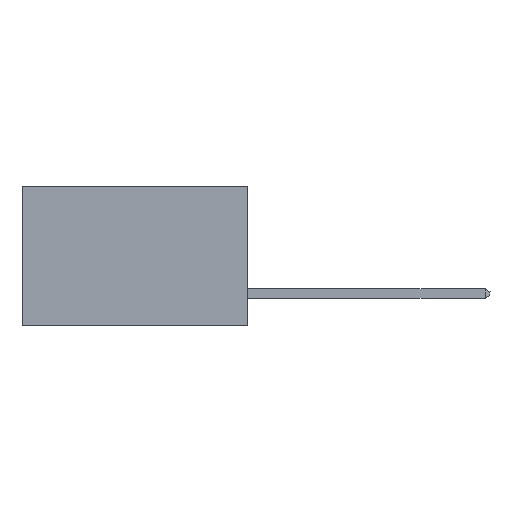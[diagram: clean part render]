
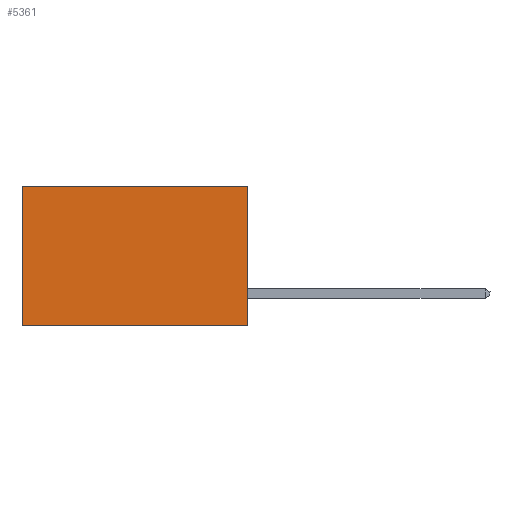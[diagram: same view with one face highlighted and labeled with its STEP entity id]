
A CAD part, left-side view. The second image highlights one B-rep face of the part: STEP entity #5361.
In plain terms, the highlighted planar face has unit normal (-1, 0, 0).
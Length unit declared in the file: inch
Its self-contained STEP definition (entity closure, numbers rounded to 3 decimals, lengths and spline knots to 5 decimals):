
#137 = EDGE_CURVE ( 'NONE', #7406, #227, #6344, .T. ) ;
#227 = VERTEX_POINT ( 'NONE', #5044 ) ;
#531 = CARTESIAN_POINT ( 'NONE',  ( 0.2615, 0.6, -0.37 ) ) ;
#715 = VECTOR ( 'NONE', #3175, 39.37008 ) ;
#822 = FACE_OUTER_BOUND ( 'NONE', #2043, .T. ) ;
#866 = VECTOR ( 'NONE', #8240, 39.37008 ) ;
#924 = ORIENTED_EDGE ( 'NONE', *, *, #137, .T. ) ;
#1146 = DIRECTION ( 'NONE',  ( 0., 1., 0. ) ) ;
#2043 = EDGE_LOOP ( 'NONE', ( #2177, #7409, #5523, #924 ) ) ;
#2177 = ORIENTED_EDGE ( 'NONE', *, *, #7890, .T. ) ;
#3007 = DIRECTION ( 'NONE',  ( 1., 0., 0. ) ) ;
#3175 = DIRECTION ( 'NONE',  ( 0., 0., -1. ) ) ;
#3201 = VECTOR ( 'NONE', #1146, 39.37008 ) ;
#4144 = CARTESIAN_POINT ( 'NONE',  ( 0.2615, 0., -0.37 ) ) ;
#4199 = VERTEX_POINT ( 'NONE', #5785 ) ;
#4618 = VECTOR ( 'NONE', #5422, 39.37008 ) ;
#5044 = CARTESIAN_POINT ( 'NONE',  ( 0.2615, 0.6, 0. ) ) ;
#5123 = CARTESIAN_POINT ( 'NONE',  ( 0.2615, 0., 0. ) ) ;
#5172 = CARTESIAN_POINT ( 'NONE',  ( 0.2615, 0., 0. ) ) ;
#5361 = ADVANCED_FACE ( 'NONE', ( #822 ), #7408, .F. ) ;
#5422 = DIRECTION ( 'NONE',  ( 0., 0., -1. ) ) ;
#5523 = ORIENTED_EDGE ( 'NONE', *, *, #6398, .F. ) ;
#5676 = CARTESIAN_POINT ( 'NONE',  ( 0.2615, 0., -0.37 ) ) ;
#5727 = LINE ( 'NONE', #5676, #3201 ) ;
#5785 = CARTESIAN_POINT ( 'NONE',  ( 0.2615, 0.6, -0.37 ) ) ;
#6250 = CARTESIAN_POINT ( 'NONE',  ( 0.2615, 0., -0.37 ) ) ;
#6344 = LINE ( 'NONE', #5123, #866 ) ;
#6398 = EDGE_CURVE ( 'NONE', #7406, #8041, #7339, .T. ) ;
#6477 = LINE ( 'NONE', #531, #715 ) ;
#6702 = CARTESIAN_POINT ( 'NONE',  ( 0.2615, 0., -0.37 ) ) ;
#7339 = LINE ( 'NONE', #6702, #4618 ) ;
#7406 = VERTEX_POINT ( 'NONE', #5172 ) ;
#7408 = PLANE ( 'NONE',  #7981 ) ;
#7409 = ORIENTED_EDGE ( 'NONE', *, *, #8115, .F. ) ;
#7449 = DIRECTION ( 'NONE',  ( 0., 0., -1. ) ) ;
#7890 = EDGE_CURVE ( 'NONE', #227, #4199, #6477, .T. ) ;
#7981 = AXIS2_PLACEMENT_3D ( 'NONE', #6250, #3007, #7449 ) ;
#8041 = VERTEX_POINT ( 'NONE', #4144 ) ;
#8115 = EDGE_CURVE ( 'NONE', #8041, #4199, #5727, .T. ) ;
#8240 = DIRECTION ( 'NONE',  ( 0., 1., 0. ) ) ;
